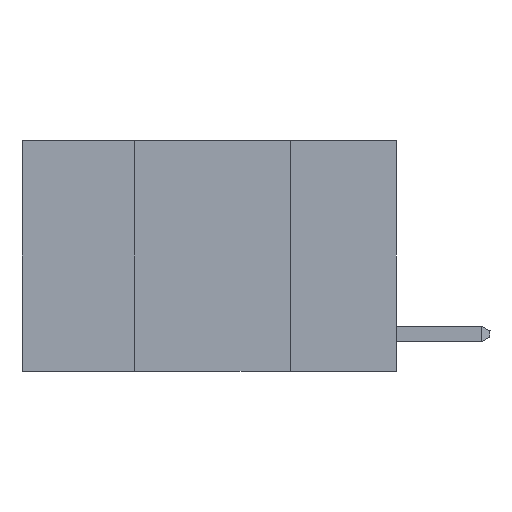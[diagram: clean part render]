
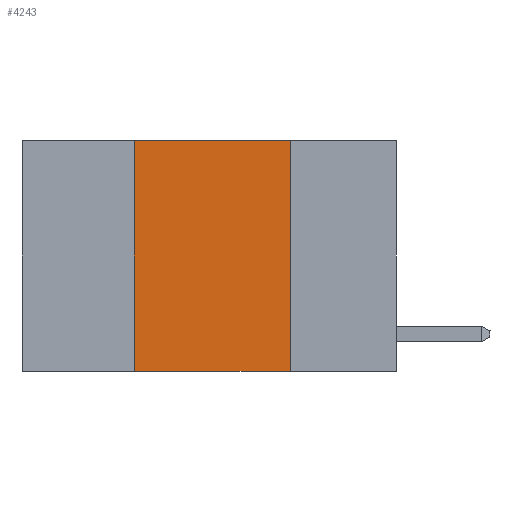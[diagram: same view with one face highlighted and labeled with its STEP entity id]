
A CAD part, left-side view. The second image highlights one B-rep face of the part: STEP entity #4243.
In plain terms, the highlighted planar face has unit normal (-1, 0, 0).
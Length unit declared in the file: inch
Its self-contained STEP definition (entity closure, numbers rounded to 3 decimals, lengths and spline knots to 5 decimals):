
#90 = LINE ( 'NONE', #10935, #12166 ) ;
#459 = ORIENTED_EDGE ( 'NONE', *, *, #758, .F. ) ;
#758 = EDGE_CURVE ( 'NONE', #6876, #10784, #4330, .T. ) ;
#813 = AXIS2_PLACEMENT_3D ( 'NONE', #7743, #4897, #11506 ) ;
#1020 = EDGE_CURVE ( 'NONE', #6308, #10784, #7742, .T. ) ;
#2691 = CARTESIAN_POINT ( 'NONE',  ( 0., 0.17, -0.37 ) ) ;
#2763 = CARTESIAN_POINT ( 'NONE',  ( 0., 0.42, 0. ) ) ;
#3788 = VERTEX_POINT ( 'NONE', #2763 ) ;
#4243 = ADVANCED_FACE ( 'NONE', ( #9440 ), #6791, .F. ) ;
#4330 = LINE ( 'NONE', #5371, #12322 ) ;
#4776 = ORIENTED_EDGE ( 'NONE', *, *, #1020, .T. ) ;
#4841 = LINE ( 'NONE', #6437, #8700 ) ;
#4897 = DIRECTION ( 'NONE',  ( 1., 0., 0. ) ) ;
#5371 = CARTESIAN_POINT ( 'NONE',  ( 0., 0.17, 0. ) ) ;
#5828 = VECTOR ( 'NONE', #7330, 39.37008 ) ;
#6308 = VERTEX_POINT ( 'NONE', #12219 ) ;
#6437 = CARTESIAN_POINT ( 'NONE',  ( 0., 0.6, 0. ) ) ;
#6791 = PLANE ( 'NONE',  #813 ) ;
#6876 = VERTEX_POINT ( 'NONE', #11474 ) ;
#7330 = DIRECTION ( 'NONE',  ( 0., -1., 0. ) ) ;
#7742 = LINE ( 'NONE', #9327, #5828 ) ;
#7743 = CARTESIAN_POINT ( 'NONE',  ( 0., 0.6, 0. ) ) ;
#8369 = ORIENTED_EDGE ( 'NONE', *, *, #11384, .F. ) ;
#8429 = DIRECTION ( 'NONE',  ( 0., -1., 0. ) ) ;
#8700 = VECTOR ( 'NONE', #8429, 39.37008 ) ;
#8718 = EDGE_CURVE ( 'NONE', #3788, #6876, #4841, .T. ) ;
#9327 = CARTESIAN_POINT ( 'NONE',  ( 0., 0.6, -0.37 ) ) ;
#9440 = FACE_OUTER_BOUND ( 'NONE', #11734, .T. ) ;
#10784 = VERTEX_POINT ( 'NONE', #2691 ) ;
#10935 = CARTESIAN_POINT ( 'NONE',  ( 0., 0.42, 0. ) ) ;
#11028 = DIRECTION ( 'NONE',  ( 0., 0., -1. ) ) ;
#11384 = EDGE_CURVE ( 'NONE', #6308, #3788, #90, .T. ) ;
#11408 = ORIENTED_EDGE ( 'NONE', *, *, #8718, .F. ) ;
#11474 = CARTESIAN_POINT ( 'NONE',  ( 0., 0.17, 0. ) ) ;
#11506 = DIRECTION ( 'NONE',  ( 0., 0., -1. ) ) ;
#11734 = EDGE_LOOP ( 'NONE', ( #459, #11408, #8369, #4776 ) ) ;
#11865 = DIRECTION ( 'NONE',  ( 0., 0., 1. ) ) ;
#12166 = VECTOR ( 'NONE', #11865, 39.37008 ) ;
#12219 = CARTESIAN_POINT ( 'NONE',  ( 0., 0.42, -0.37 ) ) ;
#12322 = VECTOR ( 'NONE', #11028, 39.37008 ) ;
